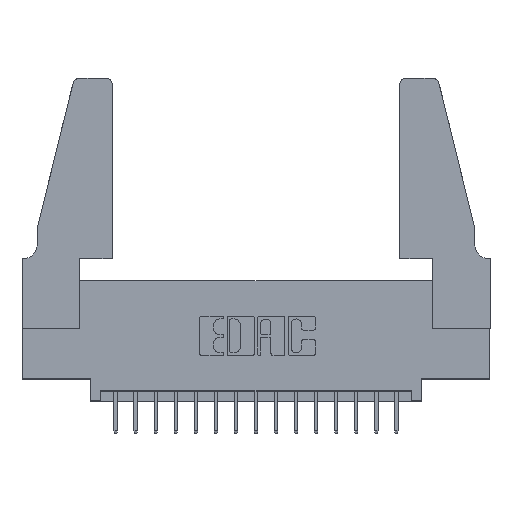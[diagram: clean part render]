
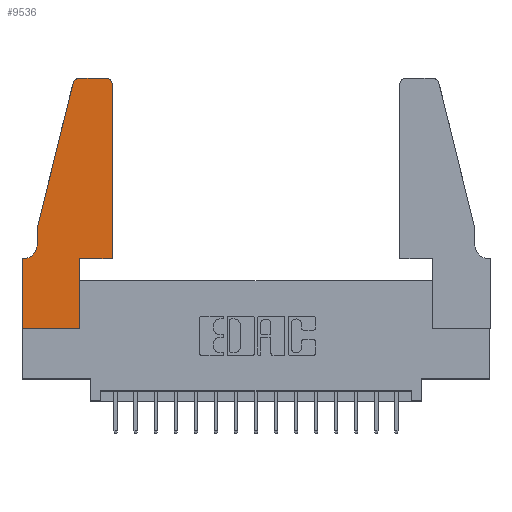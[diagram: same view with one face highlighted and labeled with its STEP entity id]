
A CAD part, top view. The second image highlights one B-rep face of the part: STEP entity #9536.
In plain terms, the highlighted planar face has unit normal (0, 0, 1).
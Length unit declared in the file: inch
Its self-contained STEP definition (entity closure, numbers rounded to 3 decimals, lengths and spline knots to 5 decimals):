
#95 = EDGE_CURVE ( 'NONE', #4710, #14433, #16360, .T. ) ;
#143 = VERTEX_POINT ( 'NONE', #9843 ) ;
#232 = DIRECTION ( 'NONE',  ( 0., 0., 1. ) ) ;
#335 = EDGE_CURVE ( 'NONE', #12920, #8217, #14417, .T. ) ;
#551 = CARTESIAN_POINT ( 'NONE',  ( 0.0755, 0.35, 0.37 ) ) ;
#815 = EDGE_CURVE ( 'NONE', #2442, #4710, #15371, .T. ) ;
#830 = AXIS2_PLACEMENT_3D ( 'NONE', #13461, #17519, #16082 ) ;
#1097 = DIRECTION ( 'NONE',  ( 0., 1., 0. ) ) ;
#1131 = ORIENTED_EDGE ( 'NONE', *, *, #14822, .T. ) ;
#1276 = EDGE_CURVE ( 'NONE', #16467, #10471, #9864, .T. ) ;
#1372 = CARTESIAN_POINT ( 'NONE',  ( 0.2865, 0.35, 0.37 ) ) ;
#1755 = ORIENTED_EDGE ( 'NONE', *, *, #95, .T. ) ;
#1844 = DIRECTION ( 'NONE',  ( 1., 0., 0. ) ) ;
#1862 = CIRCLE ( 'NONE', #9079, 0.07 ) ;
#1989 = CARTESIAN_POINT ( 'NONE',  ( 0.2605, 1.25, 0.37 ) ) ;
#2008 = ORIENTED_EDGE ( 'NONE', *, *, #7386, .T. ) ;
#2254 = LINE ( 'NONE', #7739, #8759 ) ;
#2282 = EDGE_CURVE ( 'NONE', #14433, #6880, #14898, .T. ) ;
#2442 = VERTEX_POINT ( 'NONE', #1372 ) ;
#2876 = CARTESIAN_POINT ( 'NONE',  ( 0.284, 1.25, 0.37 ) ) ;
#3328 = VERTEX_POINT ( 'NONE', #10629 ) ;
#3379 = VERTEX_POINT ( 'NONE', #2876 ) ;
#3632 = ORIENTED_EDGE ( 'NONE', *, *, #11151, .T. ) ;
#3734 = ORIENTED_EDGE ( 'NONE', *, *, #1276, .T. ) ;
#3830 = CARTESIAN_POINT ( 'NONE',  ( 0.2865, 0.35, 0.37 ) ) ;
#4282 = CARTESIAN_POINT ( 'NONE',  ( 0.4505, 0.35, 0.37 ) ) ;
#4459 = EDGE_LOOP ( 'NONE', ( #2008, #13488, #1131, #3632, #14983, #6962, #6172, #3734, #14086, #13421, #1755, #14003 ) ) ;
#4643 = DIRECTION ( 'NONE',  ( -1., 0., 0. ) ) ;
#4710 = VERTEX_POINT ( 'NONE', #7843 ) ;
#4912 = CARTESIAN_POINT ( 'NONE',  ( 0., 0.35, 0.37 ) ) ;
#5017 = CARTESIAN_POINT ( 'NONE',  ( 0.0055, 0.42, 0.37 ) ) ;
#5170 = EDGE_CURVE ( 'NONE', #3379, #14793, #11432, .T. ) ;
#5441 = DIRECTION ( 'NONE',  ( 0., 1., 0. ) ) ;
#5514 = DIRECTION ( 'NONE',  ( 0., 0., 1. ) ) ;
#6013 = DIRECTION ( 'NONE',  ( -1., 0., 0. ) ) ;
#6054 = LINE ( 'NONE', #15458, #9502 ) ;
#6057 = CARTESIAN_POINT ( 'NONE',  ( 0.25487, 1.22718, 0.37 ) ) ;
#6172 = ORIENTED_EDGE ( 'NONE', *, *, #13008, .T. ) ;
#6189 = DIRECTION ( 'NONE',  ( -0.239, -0.971, 0. ) ) ;
#6541 = EDGE_CURVE ( 'NONE', #3328, #12920, #1862, .T. ) ;
#6866 = CARTESIAN_POINT ( 'NONE',  ( 0., 0., 0.37 ) ) ;
#6880 = VERTEX_POINT ( 'NONE', #13507 ) ;
#6962 = ORIENTED_EDGE ( 'NONE', *, *, #335, .T. ) ;
#7074 = VECTOR ( 'NONE', #12862, 39.37008 ) ;
#7203 = CARTESIAN_POINT ( 'NONE',  ( 0., 0., 0.37 ) ) ;
#7386 = EDGE_CURVE ( 'NONE', #6880, #3379, #10910, .T. ) ;
#7739 = CARTESIAN_POINT ( 'NONE',  ( 0.0755, 0.5, 0.37 ) ) ;
#7795 = DIRECTION ( 'NONE',  ( 0., 0., -1. ) ) ;
#7843 = CARTESIAN_POINT ( 'NONE',  ( 0.4505, 0.35, 0.37 ) ) ;
#8217 = VERTEX_POINT ( 'NONE', #4912 ) ;
#8688 = AXIS2_PLACEMENT_3D ( 'NONE', #13668, #5514, #1844 ) ;
#8759 = VECTOR ( 'NONE', #6189, 39.37008 ) ;
#9079 = AXIS2_PLACEMENT_3D ( 'NONE', #5017, #7795, #16002 ) ;
#9502 = VECTOR ( 'NONE', #16854, 39.37008 ) ;
#9536 = ADVANCED_FACE ( 'NONE', ( #15497 ), #12142, .T. ) ;
#9647 = VECTOR ( 'NONE', #12638, 39.37008 ) ;
#9843 = CARTESIAN_POINT ( 'NONE',  ( 0.0755, 0.5, 0.37 ) ) ;
#9864 = LINE ( 'NONE', #7203, #9647 ) ;
#10471 = VERTEX_POINT ( 'NONE', #16492 ) ;
#10629 = CARTESIAN_POINT ( 'NONE',  ( 0.0755, 0.42, 0.37 ) ) ;
#10637 = VECTOR ( 'NONE', #4643, 39.37008 ) ;
#10910 = LINE ( 'NONE', #1989, #15120 ) ;
#10947 = CARTESIAN_POINT ( 'NONE',  ( 0.4505, 1.22, 0.37 ) ) ;
#11151 = EDGE_CURVE ( 'NONE', #143, #3328, #6054, .T. ) ;
#11308 = DIRECTION ( 'NONE',  ( 1., 0., 0. ) ) ;
#11432 = CIRCLE ( 'NONE', #8688, 0.03 ) ;
#11515 = CARTESIAN_POINT ( 'NONE',  ( 0., 0., 0.37 ) ) ;
#12142 = PLANE ( 'NONE',  #830 ) ;
#12288 = CARTESIAN_POINT ( 'NONE',  ( 0.0055, 0.35, 0.37 ) ) ;
#12345 = VECTOR ( 'NONE', #5441, 39.37008 ) ;
#12638 = DIRECTION ( 'NONE',  ( 1., 0., 0. ) ) ;
#12862 = DIRECTION ( 'NONE',  ( 0., -1., 0. ) ) ;
#12920 = VERTEX_POINT ( 'NONE', #12288 ) ;
#13008 = EDGE_CURVE ( 'NONE', #8217, #16467, #17733, .T. ) ;
#13421 = ORIENTED_EDGE ( 'NONE', *, *, #815, .T. ) ;
#13461 = CARTESIAN_POINT ( 'NONE',  ( 0., 0.35, 0.37 ) ) ;
#13488 = ORIENTED_EDGE ( 'NONE', *, *, #5170, .T. ) ;
#13507 = CARTESIAN_POINT ( 'NONE',  ( 0.4205, 1.25, 0.37 ) ) ;
#13668 = CARTESIAN_POINT ( 'NONE',  ( 0.284, 1.22, 0.37 ) ) ;
#14003 = ORIENTED_EDGE ( 'NONE', *, *, #2282, .T. ) ;
#14086 = ORIENTED_EDGE ( 'NONE', *, *, #15742, .T. ) ;
#14417 = LINE ( 'NONE', #551, #10637 ) ;
#14433 = VERTEX_POINT ( 'NONE', #10947 ) ;
#14779 = CARTESIAN_POINT ( 'NONE',  ( 0.4505, 0.35, 0.37 ) ) ;
#14793 = VERTEX_POINT ( 'NONE', #6057 ) ;
#14822 = EDGE_CURVE ( 'NONE', #14793, #143, #2254, .T. ) ;
#14898 = CIRCLE ( 'NONE', #16541, 0.03 ) ;
#14983 = ORIENTED_EDGE ( 'NONE', *, *, #6541, .T. ) ;
#15120 = VECTOR ( 'NONE', #6013, 39.37008 ) ;
#15371 = LINE ( 'NONE', #14779, #15579 ) ;
#15458 = CARTESIAN_POINT ( 'NONE',  ( 0.0755, 0.5, 0.37 ) ) ;
#15497 = FACE_OUTER_BOUND ( 'NONE', #4459, .T. ) ;
#15579 = VECTOR ( 'NONE', #17242, 39.37008 ) ;
#15742 = EDGE_CURVE ( 'NONE', #10471, #2442, #16827, .T. ) ;
#15945 = VECTOR ( 'NONE', #1097, 39.37008 ) ;
#16002 = DIRECTION ( 'NONE',  ( -1., 0., 0. ) ) ;
#16082 = DIRECTION ( 'NONE',  ( 1., 0., 0. ) ) ;
#16360 = LINE ( 'NONE', #4282, #12345 ) ;
#16467 = VERTEX_POINT ( 'NONE', #6866 ) ;
#16492 = CARTESIAN_POINT ( 'NONE',  ( 0.2865, 0., 0.37 ) ) ;
#16541 = AXIS2_PLACEMENT_3D ( 'NONE', #16704, #232, #11308 ) ;
#16704 = CARTESIAN_POINT ( 'NONE',  ( 0.4205, 1.22, 0.37 ) ) ;
#16827 = LINE ( 'NONE', #3830, #15945 ) ;
#16854 = DIRECTION ( 'NONE',  ( 0., -1., 0. ) ) ;
#17242 = DIRECTION ( 'NONE',  ( 1., 0., 0. ) ) ;
#17519 = DIRECTION ( 'NONE',  ( 0., 0., 1. ) ) ;
#17733 = LINE ( 'NONE', #11515, #7074 ) ;
